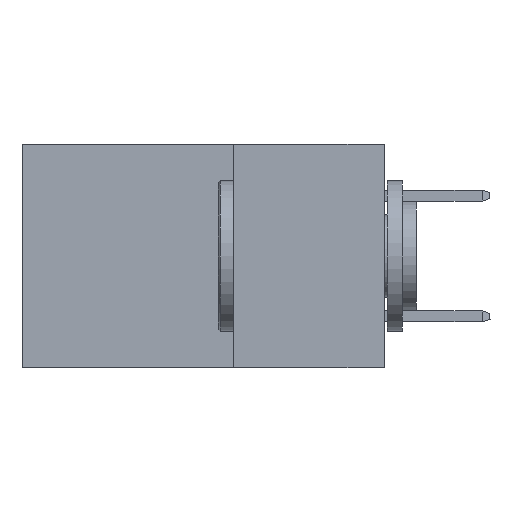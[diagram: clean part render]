
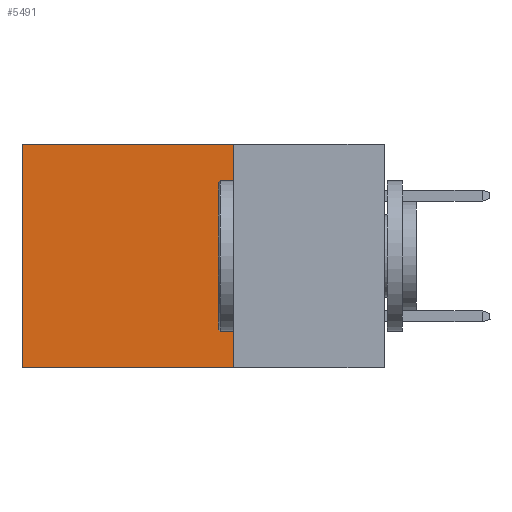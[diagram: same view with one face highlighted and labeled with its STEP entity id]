
A CAD part, left-side view. The second image highlights one B-rep face of the part: STEP entity #5491.
In plain terms, the highlighted planar face has unit normal (-1, 0, 0).
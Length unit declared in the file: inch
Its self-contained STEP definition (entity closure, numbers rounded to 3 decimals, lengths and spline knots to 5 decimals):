
#406 = VERTEX_POINT ( 'NONE', #855 ) ;
#594 = CARTESIAN_POINT ( 'NONE',  ( 0.2615, 0.25, 0. ) ) ;
#855 = CARTESIAN_POINT ( 'NONE',  ( 0.2615, 0.6, 0. ) ) ;
#885 = CARTESIAN_POINT ( 'NONE',  ( 0.2615, 0.6, -0.37 ) ) ;
#1727 = EDGE_CURVE ( 'NONE', #15019, #406, #3432, .T. ) ;
#3254 = ORIENTED_EDGE ( 'NONE', *, *, #1727, .T. ) ;
#3432 = LINE ( 'NONE', #594, #12819 ) ;
#5491 = ADVANCED_FACE ( 'NONE', ( #17773 ), #22167, .F. ) ;
#5824 = EDGE_CURVE ( 'NONE', #13693, #24781, #7400, .T. ) ;
#7400 = LINE ( 'NONE', #17942, #17879 ) ;
#8282 = LINE ( 'NONE', #10347, #23155 ) ;
#10347 = CARTESIAN_POINT ( 'NONE',  ( 0.2615, 0.6, -0.37 ) ) ;
#10882 = AXIS2_PLACEMENT_3D ( 'NONE', #22612, #22161, #22140 ) ;
#11545 = CARTESIAN_POINT ( 'NONE',  ( 0.2615, 0.25, -0.37 ) ) ;
#11590 = LINE ( 'NONE', #15186, #16095 ) ;
#12756 = DIRECTION ( 'NONE',  ( 0., 0., -1. ) ) ;
#12819 = VECTOR ( 'NONE', #20244, 39.37008 ) ;
#13693 = VERTEX_POINT ( 'NONE', #11545 ) ;
#14429 = ORIENTED_EDGE ( 'NONE', *, *, #5824, .F. ) ;
#15019 = VERTEX_POINT ( 'NONE', #16913 ) ;
#15186 = CARTESIAN_POINT ( 'NONE',  ( 0.2615, 0.25, -0.37 ) ) ;
#15884 = ORIENTED_EDGE ( 'NONE', *, *, #17652, .F. ) ;
#16095 = VECTOR ( 'NONE', #22796, 39.37008 ) ;
#16913 = CARTESIAN_POINT ( 'NONE',  ( 0.2615, 0.25, 0. ) ) ;
#17652 = EDGE_CURVE ( 'NONE', #15019, #13693, #11590, .T. ) ;
#17773 = FACE_OUTER_BOUND ( 'NONE', #19108, .T. ) ;
#17879 = VECTOR ( 'NONE', #18160, 39.37008 ) ;
#17942 = CARTESIAN_POINT ( 'NONE',  ( 0.2615, 0.25, -0.37 ) ) ;
#18160 = DIRECTION ( 'NONE',  ( 0., 1., 0. ) ) ;
#19108 = EDGE_LOOP ( 'NONE', ( #20266, #14429, #15884, #3254 ) ) ;
#20244 = DIRECTION ( 'NONE',  ( 0., 1., 0. ) ) ;
#20266 = ORIENTED_EDGE ( 'NONE', *, *, #20528, .T. ) ;
#20528 = EDGE_CURVE ( 'NONE', #406, #24781, #8282, .T. ) ;
#22140 = DIRECTION ( 'NONE',  ( 0., 0., -1. ) ) ;
#22161 = DIRECTION ( 'NONE',  ( 1., 0., 0. ) ) ;
#22167 = PLANE ( 'NONE',  #10882 ) ;
#22612 = CARTESIAN_POINT ( 'NONE',  ( 0.2615, 0.25, -0.37 ) ) ;
#22796 = DIRECTION ( 'NONE',  ( 0., 0., -1. ) ) ;
#23155 = VECTOR ( 'NONE', #12756, 39.37008 ) ;
#24781 = VERTEX_POINT ( 'NONE', #885 ) ;
